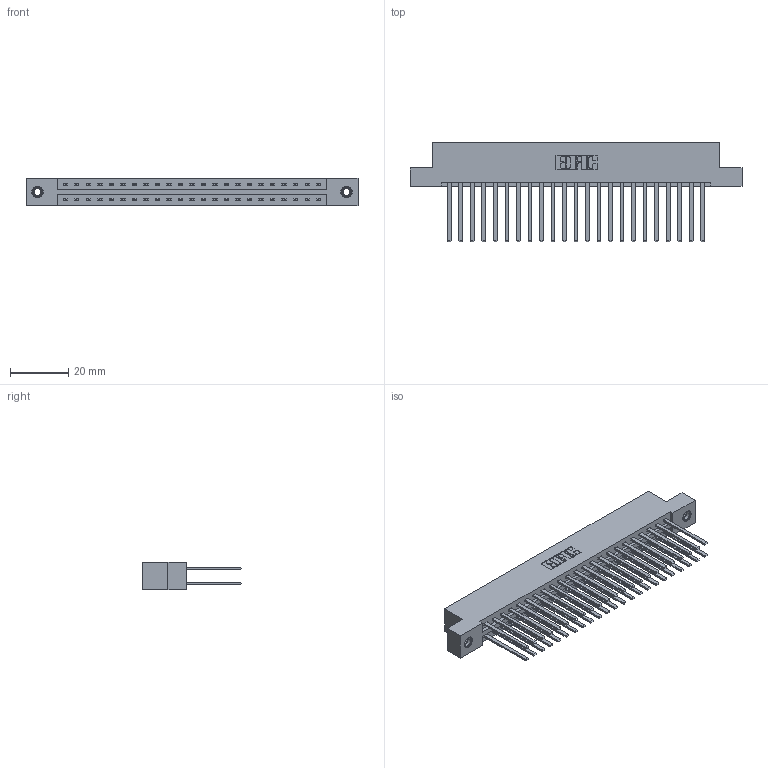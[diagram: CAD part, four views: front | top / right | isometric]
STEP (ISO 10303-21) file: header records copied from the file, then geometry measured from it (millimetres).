
FILE_DESCRIPTION (( 'STEP AP203' ), '1' );
FILE_NAME ('387-046-544-208.STEP', '2018-09-20T04:19:04', ( '' ), ( '' ), 'SwSTEP 2.0', 'SolidWorks 2016', '' );
FILE_SCHEMA (( 'CONFIG_CONTROL_DESIGN' ));
Length unit declared in the file: inch
Products named in the file (4): 337 Part_Flush Mounting Lugs - 0.156 Dia-TI; 345-292-001_345-293-144; 345-250-001_345-250-003-102; 387-046-544-208
Assembly tree (49 placements, depth 2):
  387-046-544-208
    337 Part_Flush Mounting Lugs - 0.156 Dia-TI
    345-292-001_345-293-144  x46
    345-250-001_345-250-003-102  x2
Bounding box: 114.15 x 34.3 x 9.4 mm (x, y, z)
Volume: 12415.2 mm3; surface area: 15981.3 mm2
Topology: 49 solids, 49 shells, 2382 faces, 7025 edges, 4614 vertices
Faces by surface type: plane 1666, cylinder 700, cone 12, torus 4
Entity records: 21292 total; most frequent: CARTESIAN_POINT 3581, ORIENTED_EDGE 3510, DIRECTION 3109, EDGE_CURVE 1755, LINE 1611, VECTOR 1611, VERTEX_POINT 1164, AXIS2_PLACEMENT_3D 749
